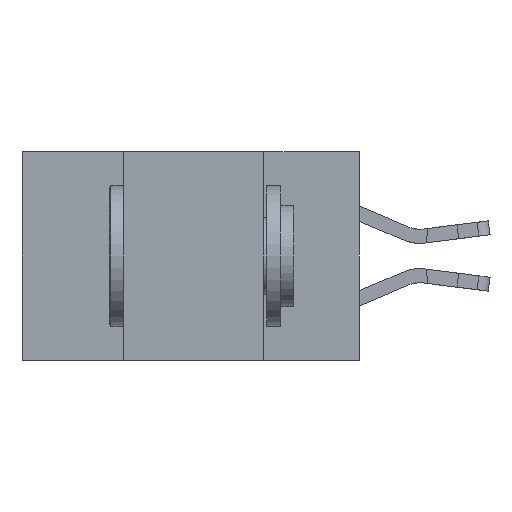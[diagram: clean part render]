
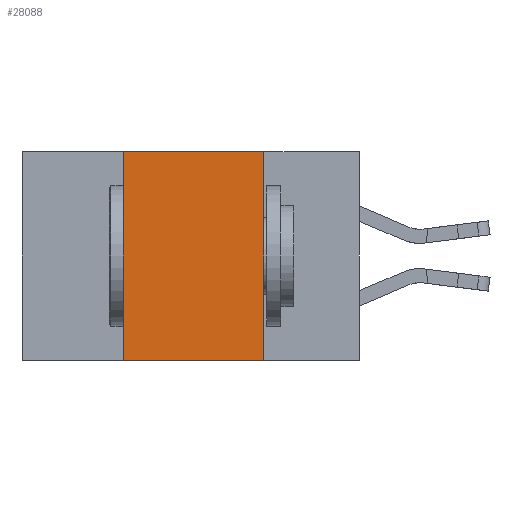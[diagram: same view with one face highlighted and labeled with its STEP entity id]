
A CAD part, left-side view. The second image highlights one B-rep face of the part: STEP entity #28088.
In plain terms, the highlighted planar face has unit normal (-1, 0, 0).
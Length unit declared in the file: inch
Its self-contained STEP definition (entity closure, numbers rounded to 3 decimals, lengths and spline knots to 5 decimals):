
#362 = LINE ( 'NONE', #8461, #22786 ) ;
#727 = EDGE_LOOP ( 'NONE', ( #6074, #4803, #26837, #9693 ) ) ;
#1234 = VERTEX_POINT ( 'NONE', #9620 ) ;
#4027 = DIRECTION ( 'NONE',  ( 0., 0., -1. ) ) ;
#4803 = ORIENTED_EDGE ( 'NONE', *, *, #16512, .F. ) ;
#5509 = CARTESIAN_POINT ( 'NONE',  ( 0., 0.17, 0. ) ) ;
#5591 = LINE ( 'NONE', #15839, #20555 ) ;
#6074 = ORIENTED_EDGE ( 'NONE', *, *, #12173, .F. ) ;
#7190 = VECTOR ( 'NONE', #27652, 39.37008 ) ;
#8461 = CARTESIAN_POINT ( 'NONE',  ( 0., 0.17, 0. ) ) ;
#8601 = CARTESIAN_POINT ( 'NONE',  ( 0., 0.6, 0. ) ) ;
#9205 = LINE ( 'NONE', #21752, #19957 ) ;
#9620 = CARTESIAN_POINT ( 'NONE',  ( 0., 0.17, -0.37 ) ) ;
#9693 = ORIENTED_EDGE ( 'NONE', *, *, #11861, .T. ) ;
#10573 = EDGE_CURVE ( 'NONE', #20827, #13597, #13552, .T. ) ;
#11702 = CARTESIAN_POINT ( 'NONE',  ( 0., 0.42, -0.37 ) ) ;
#11861 = EDGE_CURVE ( 'NONE', #20827, #1234, #5591, .T. ) ;
#12173 = EDGE_CURVE ( 'NONE', #13329, #1234, #362, .T. ) ;
#12890 = AXIS2_PLACEMENT_3D ( 'NONE', #8601, #25174, #4027 ) ;
#13329 = VERTEX_POINT ( 'NONE', #5509 ) ;
#13552 = LINE ( 'NONE', #22840, #7190 ) ;
#13597 = VERTEX_POINT ( 'NONE', #20062 ) ;
#14646 = DIRECTION ( 'NONE',  ( 0., -1., 0. ) ) ;
#15624 = DIRECTION ( 'NONE',  ( 0., 0., -1. ) ) ;
#15839 = CARTESIAN_POINT ( 'NONE',  ( 0., 0.6, -0.37 ) ) ;
#16512 = EDGE_CURVE ( 'NONE', #13597, #13329, #9205, .T. ) ;
#17303 = FACE_OUTER_BOUND ( 'NONE', #727, .T. ) ;
#19957 = VECTOR ( 'NONE', #14646, 39.37008 ) ;
#20062 = CARTESIAN_POINT ( 'NONE',  ( 0., 0.42, 0. ) ) ;
#20555 = VECTOR ( 'NONE', #27768, 39.37008 ) ;
#20827 = VERTEX_POINT ( 'NONE', #11702 ) ;
#21752 = CARTESIAN_POINT ( 'NONE',  ( 0., 0.6, 0. ) ) ;
#22786 = VECTOR ( 'NONE', #15624, 39.37008 ) ;
#22840 = CARTESIAN_POINT ( 'NONE',  ( 0., 0.42, 0. ) ) ;
#25174 = DIRECTION ( 'NONE',  ( 1., 0., 0. ) ) ;
#26837 = ORIENTED_EDGE ( 'NONE', *, *, #10573, .F. ) ;
#27480 = PLANE ( 'NONE',  #12890 ) ;
#27652 = DIRECTION ( 'NONE',  ( 0., 0., 1. ) ) ;
#27768 = DIRECTION ( 'NONE',  ( 0., -1., 0. ) ) ;
#28088 = ADVANCED_FACE ( 'NONE', ( #17303 ), #27480, .F. ) ;
